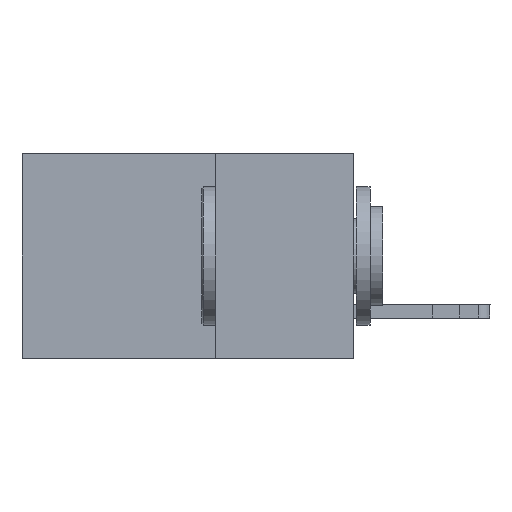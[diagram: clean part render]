
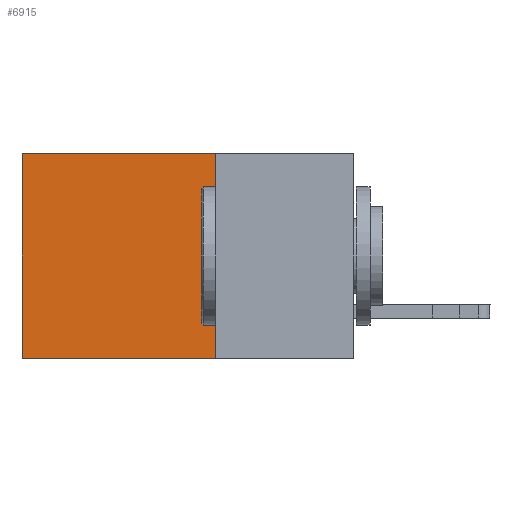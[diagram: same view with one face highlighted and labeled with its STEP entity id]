
A CAD part, left-side view. The second image highlights one B-rep face of the part: STEP entity #6915.
In plain terms, the highlighted planar face has unit normal (-1, 0, 0).
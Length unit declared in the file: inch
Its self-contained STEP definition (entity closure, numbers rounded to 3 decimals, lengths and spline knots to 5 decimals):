
#20 = VERTEX_POINT ( 'NONE', #5898 ) ;
#227 = EDGE_CURVE ( 'NONE', #1337, #20, #4314, .T. ) ;
#543 = CARTESIAN_POINT ( 'NONE',  ( 0.2875, 0.25, -0.37 ) ) ;
#596 = VECTOR ( 'NONE', #14109, 39.37008 ) ;
#612 = CARTESIAN_POINT ( 'NONE',  ( 0.2875, 0.6, -0.37 ) ) ;
#1337 = VERTEX_POINT ( 'NONE', #9533 ) ;
#1548 = DIRECTION ( 'NONE',  ( 0., 1., 0. ) ) ;
#1665 = VECTOR ( 'NONE', #1548, 39.37008 ) ;
#3920 = CARTESIAN_POINT ( 'NONE',  ( 0.2875, 0.6, 0. ) ) ;
#4050 = FACE_OUTER_BOUND ( 'NONE', #9644, .T. ) ;
#4314 = LINE ( 'NONE', #5716, #596 ) ;
#4566 = AXIS2_PLACEMENT_3D ( 'NONE', #12187, #9963, #6197 ) ;
#5681 = CARTESIAN_POINT ( 'NONE',  ( 0.2875, 0.6, 0. ) ) ;
#5716 = CARTESIAN_POINT ( 'NONE',  ( 0.2875, 0.25, 0. ) ) ;
#5898 = CARTESIAN_POINT ( 'NONE',  ( 0.2875, 0.25, -0.37 ) ) ;
#6197 = DIRECTION ( 'NONE',  ( 0., 0., -1. ) ) ;
#6556 = LINE ( 'NONE', #3920, #12023 ) ;
#6915 = ADVANCED_FACE ( 'NONE', ( #4050 ), #11143, .F. ) ;
#8665 = CARTESIAN_POINT ( 'NONE',  ( 0.2875, 0.25, 0. ) ) ;
#9533 = CARTESIAN_POINT ( 'NONE',  ( 0.2875, 0.25, 0. ) ) ;
#9537 = LINE ( 'NONE', #543, #12817 ) ;
#9644 = EDGE_LOOP ( 'NONE', ( #10283, #12765, #11565, #13605 ) ) ;
#9958 = DIRECTION ( 'NONE',  ( 0., 0., -1. ) ) ;
#9963 = DIRECTION ( 'NONE',  ( 1., 0., 0. ) ) ;
#10283 = ORIENTED_EDGE ( 'NONE', *, *, #13802, .T. ) ;
#11143 = PLANE ( 'NONE',  #4566 ) ;
#11237 = DIRECTION ( 'NONE',  ( 0., 1., 0. ) ) ;
#11415 = LINE ( 'NONE', #8665, #1665 ) ;
#11565 = ORIENTED_EDGE ( 'NONE', *, *, #227, .F. ) ;
#11625 = VERTEX_POINT ( 'NONE', #5681 ) ;
#12023 = VECTOR ( 'NONE', #9958, 39.37008 ) ;
#12129 = VERTEX_POINT ( 'NONE', #612 ) ;
#12187 = CARTESIAN_POINT ( 'NONE',  ( 0.2875, 0.25, 0. ) ) ;
#12380 = EDGE_CURVE ( 'NONE', #20, #12129, #9537, .T. ) ;
#12765 = ORIENTED_EDGE ( 'NONE', *, *, #12380, .F. ) ;
#12817 = VECTOR ( 'NONE', #11237, 39.37008 ) ;
#13605 = ORIENTED_EDGE ( 'NONE', *, *, #14955, .T. ) ;
#13802 = EDGE_CURVE ( 'NONE', #11625, #12129, #6556, .T. ) ;
#14109 = DIRECTION ( 'NONE',  ( 0., 0., -1. ) ) ;
#14955 = EDGE_CURVE ( 'NONE', #1337, #11625, #11415, .T. ) ;
